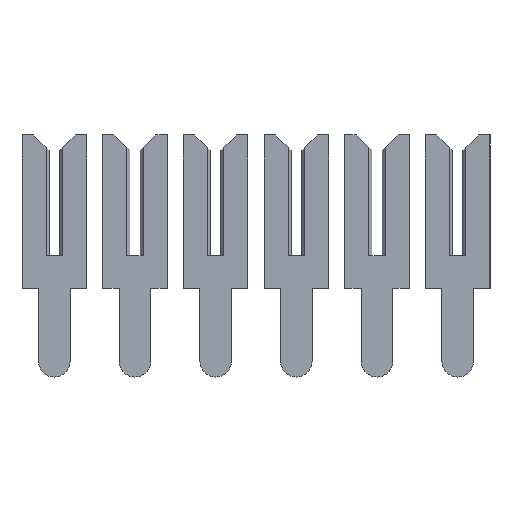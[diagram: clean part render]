
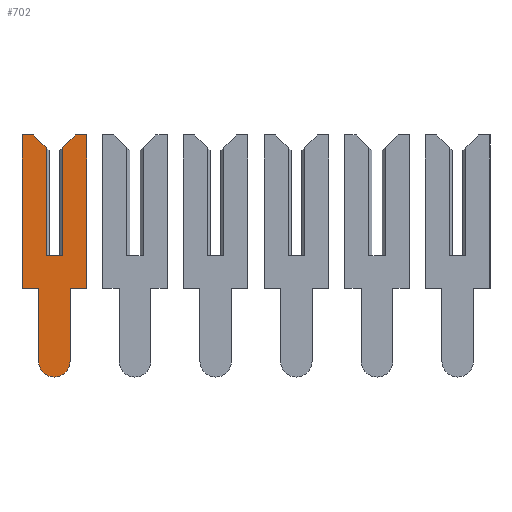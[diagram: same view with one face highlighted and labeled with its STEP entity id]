
A CAD part, top view. The second image highlights one B-rep face of the part: STEP entity #702.
In plain terms, the highlighted face is planar.
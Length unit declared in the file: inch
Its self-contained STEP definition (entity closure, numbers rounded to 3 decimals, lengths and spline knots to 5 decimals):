
#7 = ORIENTED_EDGE ( 'NONE', *, *, #232, .F. ) ;
#28 = LINE ( 'NONE', #442, #203 ) ;
#35 = CARTESIAN_POINT ( 'NONE',  ( -0.01, 0.15, 0.04 ) ) ;
#38 = DIRECTION ( 'NONE',  ( 0., -1., 0. ) ) ;
#99 = FACE_OUTER_BOUND ( 'NONE', #411, .T. ) ;
#102 = CARTESIAN_POINT ( 'NONE',  ( -0.01, -0.04, 0.0195 ) ) ;
#106 = VERTEX_POINT ( 'NONE', #146 ) ;
#108 = EDGE_CURVE ( 'NONE', #751, #334, #196, .T. ) ;
#127 = EDGE_CURVE ( 'NONE', #457, #408, #346, .T. ) ;
#135 = VERTEX_POINT ( 'NONE', #472 ) ;
#146 = CARTESIAN_POINT ( 'NONE',  ( -0.01, -0.1305, -0.0195 ) ) ;
#148 = VERTEX_POINT ( 'NONE', #615 ) ;
#155 = CARTESIAN_POINT ( 'NONE',  ( -0.01, 0., 0.01 ) ) ;
#157 = VECTOR ( 'NONE', #530, 39.37008 ) ;
#185 = CARTESIAN_POINT ( 'NONE',  ( -0.01, 0.134, 0.01 ) ) ;
#192 = LINE ( 'NONE', #270, #529 ) ;
#195 = DIRECTION ( 'NONE',  ( 1., 0., 0. ) ) ;
#196 = LINE ( 'NONE', #765, #939 ) ;
#201 = VERTEX_POINT ( 'NONE', #155 ) ;
#203 = VECTOR ( 'NONE', #820, 39.37008 ) ;
#206 = PLANE ( 'NONE',  #358 ) ;
#213 = EDGE_CURVE ( 'NONE', #469, #751, #877, .T. ) ;
#217 = ORIENTED_EDGE ( 'NONE', *, *, #425, .F. ) ;
#228 = LINE ( 'NONE', #730, #801 ) ;
#231 = DIRECTION ( 'NONE',  ( 0., 0., 1. ) ) ;
#232 = EDGE_CURVE ( 'NONE', #510, #524, #868, .T. ) ;
#234 = CARTESIAN_POINT ( 'NONE',  ( -0.01, 0., 0.0065 ) ) ;
#235 = LINE ( 'NONE', #951, #388 ) ;
#237 = EDGE_CURVE ( 'NONE', #148, #201, #978, .T. ) ;
#243 = VERTEX_POINT ( 'NONE', #318 ) ;
#252 = LINE ( 'NONE', #276, #504 ) ;
#253 = CARTESIAN_POINT ( 'NONE',  ( -0.01, -0.04, 0.04 ) ) ;
#270 = CARTESIAN_POINT ( 'NONE',  ( -0.01, 0.15, 0.026 ) ) ;
#276 = CARTESIAN_POINT ( 'NONE',  ( -0.01, 0.1305, -0.0065 ) ) ;
#283 = CARTESIAN_POINT ( 'NONE',  ( -0.01, -0.1305, 0. ) ) ;
#290 = ORIENTED_EDGE ( 'NONE', *, *, #127, .F. ) ;
#293 = ORIENTED_EDGE ( 'NONE', *, *, #108, .F. ) ;
#318 = CARTESIAN_POINT ( 'NONE',  ( -0.01, -0.1305, 0.0195 ) ) ;
#320 = DIRECTION ( 'NONE',  ( 0., 1., 0. ) ) ;
#334 = VERTEX_POINT ( 'NONE', #562 ) ;
#346 = LINE ( 'NONE', #390, #665 ) ;
#351 = DIRECTION ( 'NONE',  ( 0., -0.707, 0.707 ) ) ;
#354 = DIRECTION ( 'NONE',  ( 1., 0., 0. ) ) ;
#358 = AXIS2_PLACEMENT_3D ( 'NONE', #892, #195, #514 ) ;
#374 = ORIENTED_EDGE ( 'NONE', *, *, #439, .F. ) ;
#388 = VECTOR ( 'NONE', #869, 39.37008 ) ;
#390 = CARTESIAN_POINT ( 'NONE',  ( -0.01, 0.1305, 0.0065 ) ) ;
#392 = EDGE_CURVE ( 'NONE', #457, #201, #235, .T. ) ;
#401 = VECTOR ( 'NONE', #548, 39.37008 ) ;
#406 = VECTOR ( 'NONE', #930, 39.37008 ) ;
#408 = VERTEX_POINT ( 'NONE', #865 ) ;
#411 = EDGE_LOOP ( 'NONE', ( #976, #626, #608, #374, #293, #711, #424, #217, #926, #636, #7, #822, #647, #290 ) ) ;
#424 = ORIENTED_EDGE ( 'NONE', *, *, #742, .F. ) ;
#425 = EDGE_CURVE ( 'NONE', #106, #649, #571, .T. ) ;
#432 = DIRECTION ( 'NONE',  ( 0., 0., -1. ) ) ;
#436 = CARTESIAN_POINT ( 'NONE',  ( -0.01, -0.04, -0.0195 ) ) ;
#439 = EDGE_CURVE ( 'NONE', #334, #135, #252, .T. ) ;
#442 = CARTESIAN_POINT ( 'NONE',  ( -0.01, -0.04, -0.04 ) ) ;
#447 = LINE ( 'NONE', #35, #941 ) ;
#457 = VERTEX_POINT ( 'NONE', #185 ) ;
#469 = VERTEX_POINT ( 'NONE', #883 ) ;
#472 = CARTESIAN_POINT ( 'NONE',  ( -0.01, 0.134, -0.01 ) ) ;
#503 = DIRECTION ( 'NONE',  ( 0., 0., 1. ) ) ;
#504 = VECTOR ( 'NONE', #351, 39.37008 ) ;
#510 = VERTEX_POINT ( 'NONE', #253 ) ;
#514 = DIRECTION ( 'NONE',  ( 0., 0., -1. ) ) ;
#515 = CIRCLE ( 'NONE', #652, 0.0195 ) ;
#524 = VERTEX_POINT ( 'NONE', #102 ) ;
#528 = EDGE_CURVE ( 'NONE', #408, #914, #192, .T. ) ;
#529 = VECTOR ( 'NONE', #503, 39.37008 ) ;
#530 = DIRECTION ( 'NONE',  ( 0., -1., 0. ) ) ;
#548 = DIRECTION ( 'NONE',  ( 0., 0., -1. ) ) ;
#555 = CARTESIAN_POINT ( 'NONE',  ( -0.01, 0.15, -0.04 ) ) ;
#562 = CARTESIAN_POINT ( 'NONE',  ( -0.01, 0.15, -0.026 ) ) ;
#571 = LINE ( 'NONE', #854, #741 ) ;
#588 = DIRECTION ( 'NONE',  ( 0., -1., 0. ) ) ;
#604 = EDGE_CURVE ( 'NONE', #914, #510, #447, .T. ) ;
#608 = ORIENTED_EDGE ( 'NONE', *, *, #936, .F. ) ;
#615 = CARTESIAN_POINT ( 'NONE',  ( -0.01, 0., -0.01 ) ) ;
#623 = DIRECTION ( 'NONE',  ( 0., 0.707, 0.707 ) ) ;
#626 = ORIENTED_EDGE ( 'NONE', *, *, #237, .F. ) ;
#636 = ORIENTED_EDGE ( 'NONE', *, *, #821, .F. ) ;
#647 = ORIENTED_EDGE ( 'NONE', *, *, #528, .F. ) ;
#649 = VERTEX_POINT ( 'NONE', #436 ) ;
#652 = AXIS2_PLACEMENT_3D ( 'NONE', #283, #354, #432 ) ;
#665 = VECTOR ( 'NONE', #623, 39.37008 ) ;
#702 = ADVANCED_FACE ( 'NONE', ( #99 ), #206, .F. ) ;
#711 = ORIENTED_EDGE ( 'NONE', *, *, #213, .F. ) ;
#730 = CARTESIAN_POINT ( 'NONE',  ( -0.01, -0.04, 0.0195 ) ) ;
#741 = VECTOR ( 'NONE', #320, 39.37008 ) ;
#742 = EDGE_CURVE ( 'NONE', #649, #469, #28, .T. ) ;
#751 = VERTEX_POINT ( 'NONE', #839 ) ;
#765 = CARTESIAN_POINT ( 'NONE',  ( -0.01, 0.15, -0.026 ) ) ;
#770 = CARTESIAN_POINT ( 'NONE',  ( -0.01, -0.04, 0.04 ) ) ;
#796 = LINE ( 'NONE', #984, #157 ) ;
#801 = VECTOR ( 'NONE', #588, 39.37008 ) ;
#820 = DIRECTION ( 'NONE',  ( 0., 0., -1. ) ) ;
#821 = EDGE_CURVE ( 'NONE', #524, #243, #228, .T. ) ;
#822 = ORIENTED_EDGE ( 'NONE', *, *, #604, .F. ) ;
#839 = CARTESIAN_POINT ( 'NONE',  ( -0.01, 0.15, -0.04 ) ) ;
#840 = DIRECTION ( 'NONE',  ( 0., 0., 1. ) ) ;
#854 = CARTESIAN_POINT ( 'NONE',  ( -0.01, -0.04, -0.0195 ) ) ;
#865 = CARTESIAN_POINT ( 'NONE',  ( -0.01, 0.15, 0.026 ) ) ;
#868 = LINE ( 'NONE', #770, #401 ) ;
#869 = DIRECTION ( 'NONE',  ( 0., -1., 0. ) ) ;
#877 = LINE ( 'NONE', #555, #406 ) ;
#883 = CARTESIAN_POINT ( 'NONE',  ( -0.01, -0.04, -0.04 ) ) ;
#884 = EDGE_CURVE ( 'NONE', #243, #106, #515, .T. ) ;
#892 = CARTESIAN_POINT ( 'NONE',  ( -0.01, -0.1305, 0. ) ) ;
#903 = VECTOR ( 'NONE', #231, 39.37008 ) ;
#914 = VERTEX_POINT ( 'NONE', #972 ) ;
#926 = ORIENTED_EDGE ( 'NONE', *, *, #884, .F. ) ;
#930 = DIRECTION ( 'NONE',  ( 0., 1., 0. ) ) ;
#936 = EDGE_CURVE ( 'NONE', #135, #148, #796, .T. ) ;
#939 = VECTOR ( 'NONE', #840, 39.37008 ) ;
#941 = VECTOR ( 'NONE', #38, 39.37008 ) ;
#951 = CARTESIAN_POINT ( 'NONE',  ( -0.01, 0.15, 0.01 ) ) ;
#972 = CARTESIAN_POINT ( 'NONE',  ( -0.01, 0.15, 0.04 ) ) ;
#976 = ORIENTED_EDGE ( 'NONE', *, *, #392, .T. ) ;
#978 = LINE ( 'NONE', #234, #903 ) ;
#984 = CARTESIAN_POINT ( 'NONE',  ( -0.01, -0.1305, -0.01 ) ) ;
